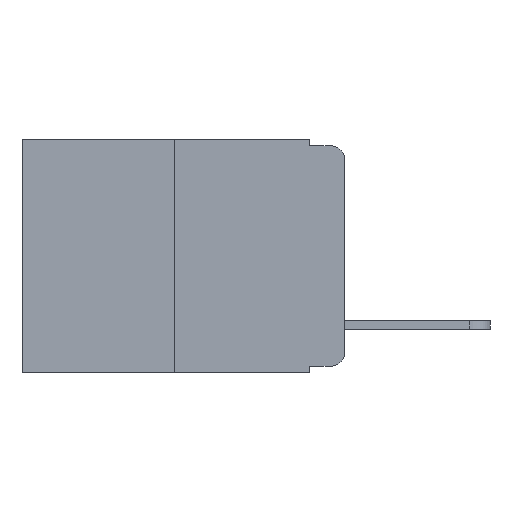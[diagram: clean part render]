
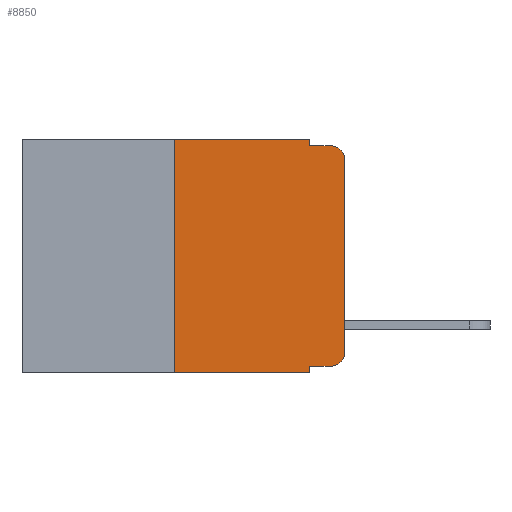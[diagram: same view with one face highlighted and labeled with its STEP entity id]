
A CAD part, left-side view. The second image highlights one B-rep face of the part: STEP entity #8850.
In plain terms, the highlighted planar face has unit normal (-1, 0, 0).
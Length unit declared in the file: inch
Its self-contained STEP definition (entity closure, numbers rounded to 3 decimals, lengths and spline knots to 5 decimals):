
#202 = EDGE_CURVE ( 'NONE', #8074, #513, #4748, .T. ) ;
#513 = VERTEX_POINT ( 'NONE', #6328 ) ;
#630 = CARTESIAN_POINT ( 'NONE',  ( 0., 0.051, 0. ) ) ;
#858 = EDGE_CURVE ( 'NONE', #5277, #513, #5434, .T. ) ;
#878 = VERTEX_POINT ( 'NONE', #1420 ) ;
#908 = EDGE_CURVE ( 'NONE', #5801, #5277, #4734, .T. ) ;
#952 = CARTESIAN_POINT ( 'NONE',  ( 0., 0.051, 0. ) ) ;
#1103 = EDGE_CURVE ( 'NONE', #4723, #11588, #8842, .T. ) ;
#1193 = DIRECTION ( 'NONE',  ( 0., 0., -1. ) ) ;
#1420 = CARTESIAN_POINT ( 'NONE',  ( 0., 0.02, -0.333 ) ) ;
#1489 = DIRECTION ( 'NONE',  ( 0., -1., 0. ) ) ;
#1607 = CARTESIAN_POINT ( 'NONE',  ( 0., 0.051, -0.01 ) ) ;
#1616 = EDGE_CURVE ( 'NONE', #2742, #9211, #8082, .T. ) ;
#1621 = LINE ( 'NONE', #10315, #6708 ) ;
#1638 = EDGE_CURVE ( 'NONE', #2742, #878, #2183, .T. ) ;
#1876 = EDGE_CURVE ( 'NONE', #878, #11592, #7648, .T. ) ;
#2144 = ORIENTED_EDGE ( 'NONE', *, *, #4776, .T. ) ;
#2183 = LINE ( 'NONE', #6573, #5084 ) ;
#2305 = DIRECTION ( 'NONE',  ( 0., 0., 1. ) ) ;
#2321 = CARTESIAN_POINT ( 'NONE',  ( 0., 0., 0. ) ) ;
#2457 = AXIS2_PLACEMENT_3D ( 'NONE', #2974, #4039, #4023 ) ;
#2537 = EDGE_LOOP ( 'NONE', ( #2144, #3152, #3153, #3293, #3324, #3360, #3657, #4736, #5723, #8076 ) ) ;
#2635 = LINE ( 'NONE', #2321, #7887 ) ;
#2742 = VERTEX_POINT ( 'NONE', #12655 ) ;
#2757 = CARTESIAN_POINT ( 'NONE',  ( 0., 0.051, -0.343 ) ) ;
#2974 = CARTESIAN_POINT ( 'NONE',  ( 0., 0.473, 0. ) ) ;
#3114 = DIRECTION ( 'NONE',  ( -1., 0., 0. ) ) ;
#3152 = ORIENTED_EDGE ( 'NONE', *, *, #202, .T. ) ;
#3153 = ORIENTED_EDGE ( 'NONE', *, *, #858, .F. ) ;
#3293 = ORIENTED_EDGE ( 'NONE', *, *, #908, .F. ) ;
#3324 = ORIENTED_EDGE ( 'NONE', *, *, #9428, .F. ) ;
#3360 = ORIENTED_EDGE ( 'NONE', *, *, #1103, .F. ) ;
#3373 = PLANE ( 'NONE',  #2457 ) ;
#3535 = DIRECTION ( 'NONE',  ( 0., -1., 0. ) ) ;
#3616 = CARTESIAN_POINT ( 'NONE',  ( 0., 0.473, -0.343 ) ) ;
#3657 = ORIENTED_EDGE ( 'NONE', *, *, #12627, .T. ) ;
#3753 = FACE_OUTER_BOUND ( 'NONE', #2537, .T. ) ;
#4023 = DIRECTION ( 'NONE',  ( 0., 0., -1. ) ) ;
#4039 = DIRECTION ( 'NONE',  ( 1., 0., 0. ) ) ;
#4050 = CARTESIAN_POINT ( 'NONE',  ( 0., 0., -0.03 ) ) ;
#4723 = VERTEX_POINT ( 'NONE', #11806 ) ;
#4734 = LINE ( 'NONE', #952, #11989 ) ;
#4736 = ORIENTED_EDGE ( 'NONE', *, *, #1616, .F. ) ;
#4748 = CIRCLE ( 'NONE', #12403, 0.02 ) ;
#4776 = EDGE_CURVE ( 'NONE', #11592, #8074, #2635, .T. ) ;
#5084 = VECTOR ( 'NONE', #10807, 39.37008 ) ;
#5277 = VERTEX_POINT ( 'NONE', #6884 ) ;
#5434 = LINE ( 'NONE', #1607, #5793 ) ;
#5525 = CARTESIAN_POINT ( 'NONE',  ( 0., 0.25, 0. ) ) ;
#5718 = LINE ( 'NONE', #3616, #10480 ) ;
#5723 = ORIENTED_EDGE ( 'NONE', *, *, #1638, .T. ) ;
#5793 = VECTOR ( 'NONE', #1489, 39.37008 ) ;
#5801 = VERTEX_POINT ( 'NONE', #10608 ) ;
#5842 = DIRECTION ( 'NONE',  ( 0., 0., 1. ) ) ;
#5958 = VECTOR ( 'NONE', #5842, 39.37008 ) ;
#6328 = CARTESIAN_POINT ( 'NONE',  ( 0., 0.02, -0.01 ) ) ;
#6573 = CARTESIAN_POINT ( 'NONE',  ( 0., 0.051, -0.333 ) ) ;
#6708 = VECTOR ( 'NONE', #10411, 39.37008 ) ;
#6884 = CARTESIAN_POINT ( 'NONE',  ( 0., 0.051, -0.01 ) ) ;
#6892 = DIRECTION ( 'NONE',  ( 0., 0., -1. ) ) ;
#7648 = CIRCLE ( 'NONE', #8556, 0.02 ) ;
#7887 = VECTOR ( 'NONE', #2305, 39.37008 ) ;
#8074 = VERTEX_POINT ( 'NONE', #4050 ) ;
#8076 = ORIENTED_EDGE ( 'NONE', *, *, #1876, .T. ) ;
#8082 = LINE ( 'NONE', #630, #10271 ) ;
#8519 = CARTESIAN_POINT ( 'NONE',  ( 0., 0.02, -0.313 ) ) ;
#8556 = AXIS2_PLACEMENT_3D ( 'NONE', #8519, #3114, #6892 ) ;
#8842 = LINE ( 'NONE', #5525, #5958 ) ;
#8850 = ADVANCED_FACE ( 'NONE', ( #3753 ), #3373, .F. ) ;
#9211 = VERTEX_POINT ( 'NONE', #2757 ) ;
#9425 = CARTESIAN_POINT ( 'NONE',  ( 0., 0.25, 0. ) ) ;
#9428 = EDGE_CURVE ( 'NONE', #11588, #5801, #1621, .T. ) ;
#9435 = CARTESIAN_POINT ( 'NONE',  ( 0., 0., -0.313 ) ) ;
#9492 = DIRECTION ( 'NONE',  ( 0., 0., -1. ) ) ;
#9521 = DIRECTION ( 'NONE',  ( -1., 0., 0. ) ) ;
#9536 = CARTESIAN_POINT ( 'NONE',  ( 0., 0.02, -0.03 ) ) ;
#10271 = VECTOR ( 'NONE', #11418, 39.37008 ) ;
#10315 = CARTESIAN_POINT ( 'NONE',  ( 0., 0.473, 0. ) ) ;
#10411 = DIRECTION ( 'NONE',  ( 0., -1., 0. ) ) ;
#10480 = VECTOR ( 'NONE', #3535, 39.37008 ) ;
#10608 = CARTESIAN_POINT ( 'NONE',  ( 0., 0.051, 0. ) ) ;
#10807 = DIRECTION ( 'NONE',  ( 0., -1., 0. ) ) ;
#11418 = DIRECTION ( 'NONE',  ( 0., 0., -1. ) ) ;
#11588 = VERTEX_POINT ( 'NONE', #9425 ) ;
#11592 = VERTEX_POINT ( 'NONE', #9435 ) ;
#11806 = CARTESIAN_POINT ( 'NONE',  ( 0., 0.25, -0.343 ) ) ;
#11989 = VECTOR ( 'NONE', #1193, 39.37008 ) ;
#12403 = AXIS2_PLACEMENT_3D ( 'NONE', #9536, #9521, #9492 ) ;
#12627 = EDGE_CURVE ( 'NONE', #4723, #9211, #5718, .T. ) ;
#12655 = CARTESIAN_POINT ( 'NONE',  ( 0., 0.051, -0.333 ) ) ;
